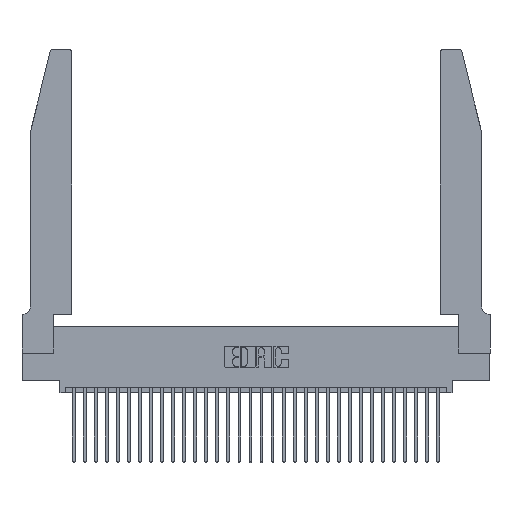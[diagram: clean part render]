
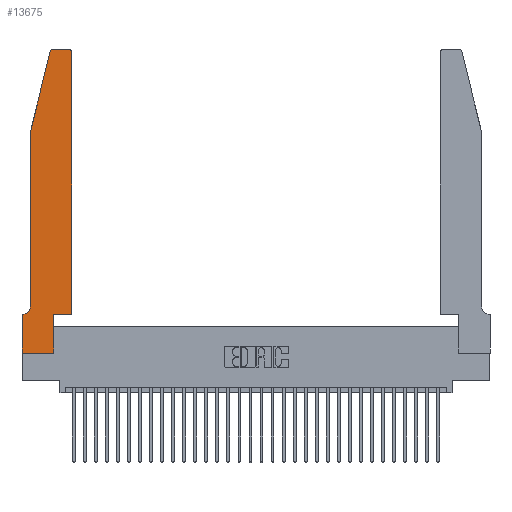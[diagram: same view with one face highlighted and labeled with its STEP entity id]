
A CAD part, top view. The second image highlights one B-rep face of the part: STEP entity #13675.
In plain terms, the highlighted planar face has unit normal (0, 0, 1).
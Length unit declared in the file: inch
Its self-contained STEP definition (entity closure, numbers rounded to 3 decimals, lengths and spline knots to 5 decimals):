
#25 = ORIENTED_EDGE ( 'NONE', *, *, #30027, .T. ) ;
#92 = DIRECTION ( 'NONE',  ( -1., 0., 0. ) ) ;
#1035 = DIRECTION ( 'NONE',  ( 0., 1., 0. ) ) ;
#1152 = VECTOR ( 'NONE', #1035, 39.37008 ) ;
#1697 = EDGE_CURVE ( 'NONE', #26079, #8238, #8422, .T. ) ;
#2049 = AXIS2_PLACEMENT_3D ( 'NONE', #27422, #15057, #4658 ) ;
#2746 = EDGE_CURVE ( 'NONE', #31455, #3233, #27366, .T. ) ;
#2988 = DIRECTION ( 'NONE',  ( -1., 0., 0. ) ) ;
#3079 = VECTOR ( 'NONE', #9104, 39.37008 ) ;
#3233 = VERTEX_POINT ( 'NONE', #29563 ) ;
#3470 = LINE ( 'NONE', #19190, #3079 ) ;
#3488 = ORIENTED_EDGE ( 'NONE', *, *, #9494, .T. ) ;
#3864 = EDGE_CURVE ( 'NONE', #12762, #6124, #31638, .T. ) ;
#4239 = VERTEX_POINT ( 'NONE', #24169 ) ;
#4321 = CARTESIAN_POINT ( 'NONE',  ( 0.0055, 0.35, 0.37 ) ) ;
#4658 = DIRECTION ( 'NONE',  ( 1., 0., 0. ) ) ;
#4957 = EDGE_CURVE ( 'NONE', #7371, #14428, #27210, .T. ) ;
#5271 = CARTESIAN_POINT ( 'NONE',  ( 0.4505, 0.35, 0.37 ) ) ;
#5275 = ORIENTED_EDGE ( 'NONE', *, *, #4957, .T. ) ;
#5991 = DIRECTION ( 'NONE',  ( 1., 0., 0. ) ) ;
#6124 = VERTEX_POINT ( 'NONE', #9626 ) ;
#6265 = CIRCLE ( 'NONE', #24764, 0.03 ) ;
#6948 = VERTEX_POINT ( 'NONE', #26840 ) ;
#7049 = VECTOR ( 'NONE', #8025, 39.37008 ) ;
#7225 = ORIENTED_EDGE ( 'NONE', *, *, #9140, .T. ) ;
#7371 = VERTEX_POINT ( 'NONE', #20490 ) ;
#7673 = LINE ( 'NONE', #26190, #19293 ) ;
#7944 = VECTOR ( 'NONE', #29521, 39.37008 ) ;
#8025 = DIRECTION ( 'NONE',  ( 1., 0., 0. ) ) ;
#8172 = DIRECTION ( 'NONE',  ( 0., -1., 0. ) ) ;
#8238 = VERTEX_POINT ( 'NONE', #25209 ) ;
#8292 = ORIENTED_EDGE ( 'NONE', *, *, #12793, .T. ) ;
#8422 = LINE ( 'NONE', #30692, #32193 ) ;
#9100 = ORIENTED_EDGE ( 'NONE', *, *, #2746, .T. ) ;
#9104 = DIRECTION ( 'NONE',  ( 0., -1., 0. ) ) ;
#9140 = EDGE_CURVE ( 'NONE', #6948, #7371, #13785, .T. ) ;
#9163 = EDGE_CURVE ( 'NONE', #26805, #17429, #6265, .T. ) ;
#9494 = EDGE_CURVE ( 'NONE', #4239, #26805, #7673, .T. ) ;
#9626 = CARTESIAN_POINT ( 'NONE',  ( 0.0755, 0.42, 0.37 ) ) ;
#9790 = CARTESIAN_POINT ( 'NONE',  ( 0., 0., 0.37 ) ) ;
#10124 = FACE_OUTER_BOUND ( 'NONE', #20567, .T. ) ;
#11430 = VECTOR ( 'NONE', #8172, 39.37008 ) ;
#11976 = LINE ( 'NONE', #19204, #22633 ) ;
#12529 = CIRCLE ( 'NONE', #13154, 0.07 ) ;
#12762 = VERTEX_POINT ( 'NONE', #22329 ) ;
#12793 = EDGE_CURVE ( 'NONE', #14428, #4239, #28008, .T. ) ;
#13049 = EDGE_CURVE ( 'NONE', #3233, #6948, #26397, .T. ) ;
#13154 = AXIS2_PLACEMENT_3D ( 'NONE', #15195, #25670, #92 ) ;
#13231 = ORIENTED_EDGE ( 'NONE', *, *, #1697, .T. ) ;
#13628 = PLANE ( 'NONE',  #15232 ) ;
#13675 = ADVANCED_FACE ( 'NONE', ( #10124 ), #13628, .T. ) ;
#13785 = LINE ( 'NONE', #5271, #7049 ) ;
#13917 = ORIENTED_EDGE ( 'NONE', *, *, #9163, .T. ) ;
#14428 = VERTEX_POINT ( 'NONE', #25834 ) ;
#14483 = DIRECTION ( 'NONE',  ( 0., 1., 0. ) ) ;
#15057 = DIRECTION ( 'NONE',  ( 0., 0., 1. ) ) ;
#15195 = CARTESIAN_POINT ( 'NONE',  ( 0.0055, 0.42, 0.37 ) ) ;
#15232 = AXIS2_PLACEMENT_3D ( 'NONE', #15854, #16196, #5991 ) ;
#15430 = ORIENTED_EDGE ( 'NONE', *, *, #30236, .T. ) ;
#15854 = CARTESIAN_POINT ( 'NONE',  ( 0., 0.35, 0.37 ) ) ;
#16128 = VECTOR ( 'NONE', #14483, 39.37008 ) ;
#16196 = DIRECTION ( 'NONE',  ( 0., 0., 1. ) ) ;
#16245 = CARTESIAN_POINT ( 'NONE',  ( 0.284, 2.72, 0.37 ) ) ;
#17429 = VERTEX_POINT ( 'NONE', #27963 ) ;
#18886 = DIRECTION ( 'NONE',  ( 1., 0., 0. ) ) ;
#19190 = CARTESIAN_POINT ( 'NONE',  ( 0., 0., 0.37 ) ) ;
#19204 = CARTESIAN_POINT ( 'NONE',  ( 0.0755, 2., 0.37 ) ) ;
#19293 = VECTOR ( 'NONE', #21338, 39.37008 ) ;
#20375 = EDGE_CURVE ( 'NONE', #17429, #12762, #11976, .T. ) ;
#20490 = CARTESIAN_POINT ( 'NONE',  ( 0.4505, 0.35, 0.37 ) ) ;
#20567 = EDGE_LOOP ( 'NONE', ( #3488, #13917, #21073, #21820, #15430, #13231, #25, #9100, #23627, #7225, #5275, #8292 ) ) ;
#21073 = ORIENTED_EDGE ( 'NONE', *, *, #20375, .T. ) ;
#21338 = DIRECTION ( 'NONE',  ( -1., 0., 0. ) ) ;
#21820 = ORIENTED_EDGE ( 'NONE', *, *, #3864, .T. ) ;
#22329 = CARTESIAN_POINT ( 'NONE',  ( 0.0755, 2., 0.37 ) ) ;
#22633 = VECTOR ( 'NONE', #24081, 39.37008 ) ;
#23627 = ORIENTED_EDGE ( 'NONE', *, *, #13049, .T. ) ;
#24081 = DIRECTION ( 'NONE',  ( -0.239, -0.971, 0. ) ) ;
#24169 = CARTESIAN_POINT ( 'NONE',  ( 0.4205, 2.75, 0.37 ) ) ;
#24764 = AXIS2_PLACEMENT_3D ( 'NONE', #16245, #31259, #18886 ) ;
#25209 = CARTESIAN_POINT ( 'NONE',  ( 0., 0.35, 0.37 ) ) ;
#25670 = DIRECTION ( 'NONE',  ( 0., 0., -1. ) ) ;
#25834 = CARTESIAN_POINT ( 'NONE',  ( 0.4505, 2.72, 0.37 ) ) ;
#26079 = VERTEX_POINT ( 'NONE', #4321 ) ;
#26190 = CARTESIAN_POINT ( 'NONE',  ( 0.2605, 2.75, 0.37 ) ) ;
#26397 = LINE ( 'NONE', #31253, #1152 ) ;
#26745 = CARTESIAN_POINT ( 'NONE',  ( 0.4505, 0.35, 0.37 ) ) ;
#26805 = VERTEX_POINT ( 'NONE', #29780 ) ;
#26840 = CARTESIAN_POINT ( 'NONE',  ( 0.2865, 0.35, 0.37 ) ) ;
#27210 = LINE ( 'NONE', #26745, #16128 ) ;
#27366 = LINE ( 'NONE', #31865, #7944 ) ;
#27422 = CARTESIAN_POINT ( 'NONE',  ( 0.4205, 2.72, 0.37 ) ) ;
#27572 = CARTESIAN_POINT ( 'NONE',  ( 0.0755, 2., 0.37 ) ) ;
#27963 = CARTESIAN_POINT ( 'NONE',  ( 0.25487, 2.72718, 0.37 ) ) ;
#28008 = CIRCLE ( 'NONE', #2049, 0.03 ) ;
#29521 = DIRECTION ( 'NONE',  ( 1., 0., 0. ) ) ;
#29563 = CARTESIAN_POINT ( 'NONE',  ( 0.2865, 0., 0.37 ) ) ;
#29780 = CARTESIAN_POINT ( 'NONE',  ( 0.284, 2.75, 0.37 ) ) ;
#30027 = EDGE_CURVE ( 'NONE', #8238, #31455, #3470, .T. ) ;
#30236 = EDGE_CURVE ( 'NONE', #6124, #26079, #12529, .T. ) ;
#30692 = CARTESIAN_POINT ( 'NONE',  ( 0.0755, 0.35, 0.37 ) ) ;
#31253 = CARTESIAN_POINT ( 'NONE',  ( 0.2865, 0.35, 0.37 ) ) ;
#31259 = DIRECTION ( 'NONE',  ( 0., 0., 1. ) ) ;
#31455 = VERTEX_POINT ( 'NONE', #9790 ) ;
#31638 = LINE ( 'NONE', #27572, #11430 ) ;
#31865 = CARTESIAN_POINT ( 'NONE',  ( 0., 0., 0.37 ) ) ;
#32193 = VECTOR ( 'NONE', #2988, 39.37008 ) ;
